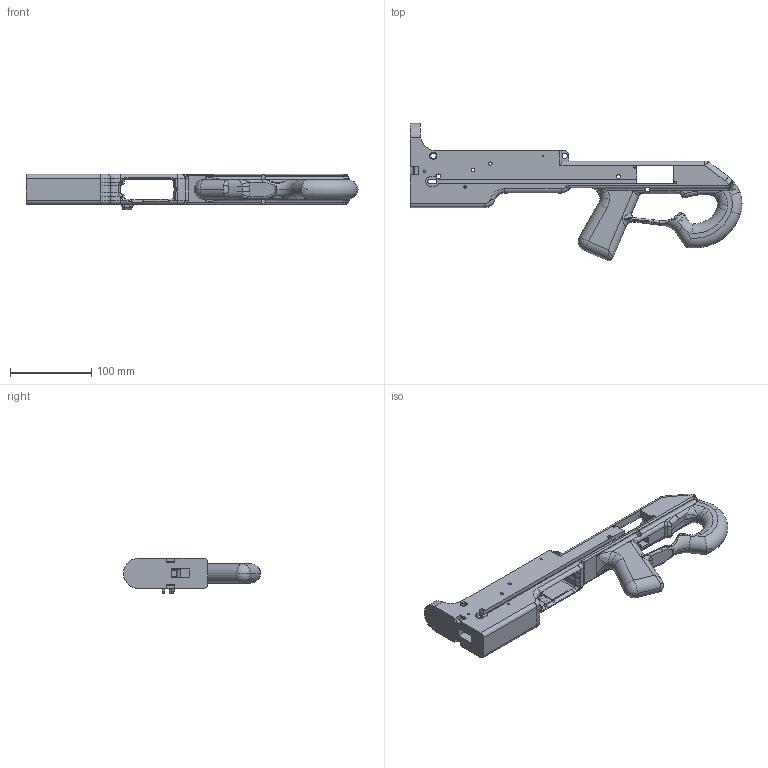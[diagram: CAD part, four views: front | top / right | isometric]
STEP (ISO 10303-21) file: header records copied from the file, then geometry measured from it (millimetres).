
FILE_DESCRIPTION (( 'STEP AP214' ), '1' );
FILE_NAME ('Hanuman_Receiver_Complete.step', '2014-05-14T06:09:56', ( 'WarFairy' ), ( '' ), 'SwSTEP 2.0', 'SolidWorks 2013', '' );
FILE_SCHEMA (( 'AUTOMOTIVE_DESIGN' ));
Length unit declared in the file: inch
Products named in the file (1): Hanuman_Receiver_Complete
Bounding box: 409.63 x 169.26 x 43.48 mm (x, y, z)
Volume: 646724.7 mm3; surface area: 127284.1 mm2
Topology: 1 solids, 1 shells, 604 faces, 1608 edges, 978 vertices
Faces by surface type: cylinder 225, plane 209, bspline 94, torus 50, cone 15, sphere 11
Entity records: 25825 total; most frequent: CARTESIAN_POINT 11452, ORIENTED_EDGE 3152, DIRECTION 2853, EDGE_CURVE 1576, AXIS2_PLACEMENT_3D 1049, VERTEX_POINT 978, VECTOR 755, LINE 755
